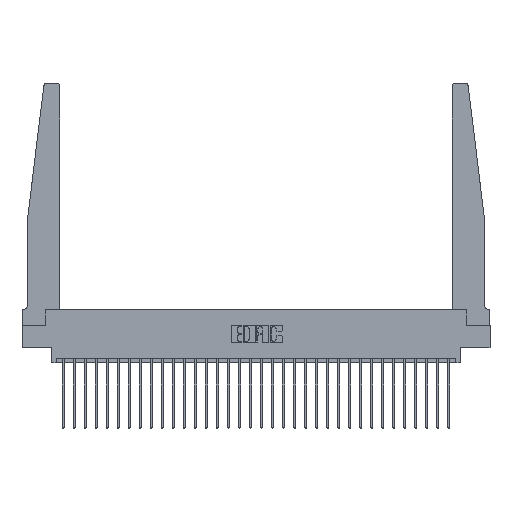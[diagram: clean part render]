
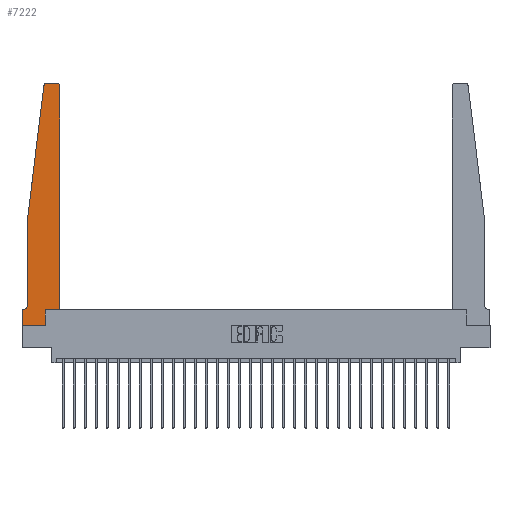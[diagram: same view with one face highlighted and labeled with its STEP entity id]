
A CAD part, top view. The second image highlights one B-rep face of the part: STEP entity #7222.
In plain terms, the highlighted planar face has unit normal (0, 0, 1).
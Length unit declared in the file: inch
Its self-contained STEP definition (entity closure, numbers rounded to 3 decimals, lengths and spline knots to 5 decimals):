
#623 = ORIENTED_EDGE ( 'NONE', *, *, #6422, .T. ) ;
#685 = VERTEX_POINT ( 'NONE', #13505 ) ;
#818 = LINE ( 'NONE', #10123, #12082 ) ;
#1288 = DIRECTION ( 'NONE',  ( 0., -1., 0. ) ) ;
#1533 = ORIENTED_EDGE ( 'NONE', *, *, #24384, .T. ) ;
#1817 = CIRCLE ( 'NONE', #18582, 0.03 ) ;
#1998 = DIRECTION ( 'NONE',  ( 1., 0., 0. ) ) ;
#2332 = LINE ( 'NONE', #20511, #6944 ) ;
#2433 = CARTESIAN_POINT ( 'NONE',  ( 0., 0., 0.37 ) ) ;
#2661 = DIRECTION ( 'NONE',  ( 1., 0., 0. ) ) ;
#2809 = FACE_OUTER_BOUND ( 'NONE', #19211, .T. ) ;
#3032 = CARTESIAN_POINT ( 'NONE',  ( 0.015, 0.1875, 0.37 ) ) ;
#3079 = CARTESIAN_POINT ( 'NONE',  ( 0., 0., 0.37 ) ) ;
#3951 = EDGE_CURVE ( 'NONE', #685, #27609, #2332, .T. ) ;
#4059 = VERTEX_POINT ( 'NONE', #3079 ) ;
#4122 = DIRECTION ( 'NONE',  ( -1., 0., 0. ) ) ;
#5247 = CARTESIAN_POINT ( 'NONE',  ( 0.2605, 0., 0.37 ) ) ;
#5410 = LINE ( 'NONE', #14570, #5514 ) ;
#5513 = VERTEX_POINT ( 'NONE', #26026 ) ;
#5514 = VECTOR ( 'NONE', #23733, 39.37008 ) ;
#5609 = VERTEX_POINT ( 'NONE', #5247 ) ;
#6367 = LINE ( 'NONE', #15544, #20562 ) ;
#6422 = EDGE_CURVE ( 'NONE', #4059, #5609, #15816, .T. ) ;
#6500 = VERTEX_POINT ( 'NONE', #21062 ) ;
#6533 = VERTEX_POINT ( 'NONE', #3032 ) ;
#6812 = CARTESIAN_POINT ( 'NONE',  ( 0.25, 2.75, 0.37 ) ) ;
#6944 = VECTOR ( 'NONE', #13451, 39.37008 ) ;
#6950 = VECTOR ( 'NONE', #1288, 39.37008 ) ;
#7222 = ADVANCED_FACE ( 'NONE', ( #2809 ), #25503, .T. ) ;
#7933 = CARTESIAN_POINT ( 'NONE',  ( 0.2605, 0.18, 0.37 ) ) ;
#7963 = CARTESIAN_POINT ( 'NONE',  ( 0.425, 2.72, 0.37 ) ) ;
#8093 = EDGE_CURVE ( 'NONE', #5513, #685, #28529, .T. ) ;
#8184 = CARTESIAN_POINT ( 'NONE',  ( 0.065, 0.2375, 0.37 ) ) ;
#8297 = EDGE_CURVE ( 'NONE', #27609, #17350, #5410, .T. ) ;
#8595 = DIRECTION ( 'NONE',  ( -1., 0., 0. ) ) ;
#10123 = CARTESIAN_POINT ( 'NONE',  ( 0.425, 0.18, 0.37 ) ) ;
#10318 = ORIENTED_EDGE ( 'NONE', *, *, #13148, .T. ) ;
#10766 = AXIS2_PLACEMENT_3D ( 'NONE', #13682, #22851, #11137 ) ;
#11137 = DIRECTION ( 'NONE',  ( 1., 0., 0. ) ) ;
#11193 = LINE ( 'NONE', #6812, #13063 ) ;
#12082 = VECTOR ( 'NONE', #21400, 39.37008 ) ;
#12377 = ORIENTED_EDGE ( 'NONE', *, *, #8297, .T. ) ;
#12617 = DIRECTION ( 'NONE',  ( 0., 1., 0. ) ) ;
#13063 = VECTOR ( 'NONE', #29522, 39.37008 ) ;
#13087 = ORIENTED_EDGE ( 'NONE', *, *, #17600, .T. ) ;
#13148 = EDGE_CURVE ( 'NONE', #25387, #23842, #818, .T. ) ;
#13277 = DIRECTION ( 'NONE',  ( 1., 0., 0. ) ) ;
#13393 = EDGE_CURVE ( 'NONE', #17350, #6533, #25638, .T. ) ;
#13451 = DIRECTION ( 'NONE',  ( -0.122, -0.992, 0. ) ) ;
#13505 = CARTESIAN_POINT ( 'NONE',  ( 0.24675, 2.72367, 0.37 ) ) ;
#13682 = CARTESIAN_POINT ( 'NONE',  ( 0.27653, 2.72, 0.37 ) ) ;
#13725 = LINE ( 'NONE', #17780, #23103 ) ;
#13769 = EDGE_CURVE ( 'NONE', #5609, #25765, #26892, .T. ) ;
#14570 = CARTESIAN_POINT ( 'NONE',  ( 0.065, 1.25, 0.37 ) ) ;
#15544 = CARTESIAN_POINT ( 'NONE',  ( 0.065, 0.1875, 0.37 ) ) ;
#15816 = LINE ( 'NONE', #2433, #24557 ) ;
#15953 = AXIS2_PLACEMENT_3D ( 'NONE', #23390, #16649, #2661 ) ;
#16202 = EDGE_CURVE ( 'NONE', #6533, #23218, #6367, .T. ) ;
#16649 = DIRECTION ( 'NONE',  ( 0., 0., 1. ) ) ;
#17350 = VERTEX_POINT ( 'NONE', #8184 ) ;
#17600 = EDGE_CURVE ( 'NONE', #6500, #5513, #11193, .T. ) ;
#17780 = CARTESIAN_POINT ( 'NONE',  ( 0.425, 0.18, 0.37 ) ) ;
#18212 = CARTESIAN_POINT ( 'NONE',  ( 0., 0.1875, 0.37 ) ) ;
#18582 = AXIS2_PLACEMENT_3D ( 'NONE', #22870, #23448, #20751 ) ;
#18937 = VECTOR ( 'NONE', #12617, 39.37008 ) ;
#19014 = EDGE_CURVE ( 'NONE', #23218, #4059, #26529, .T. ) ;
#19211 = EDGE_LOOP ( 'NONE', ( #13087, #21166, #28892, #12377, #21195, #19652, #26592, #623, #19559, #1533, #10318, #29486 ) ) ;
#19559 = ORIENTED_EDGE ( 'NONE', *, *, #13769, .T. ) ;
#19652 = ORIENTED_EDGE ( 'NONE', *, *, #16202, .T. ) ;
#20159 = CARTESIAN_POINT ( 'NONE',  ( 0.015, 0.2375, 0.37 ) ) ;
#20410 = CARTESIAN_POINT ( 'NONE',  ( 0.425, 0.18, 0.37 ) ) ;
#20511 = CARTESIAN_POINT ( 'NONE',  ( 0.065, 1.25, 0.37 ) ) ;
#20562 = VECTOR ( 'NONE', #4122, 39.37008 ) ;
#20751 = DIRECTION ( 'NONE',  ( 1., 0., 0. ) ) ;
#21062 = CARTESIAN_POINT ( 'NONE',  ( 0.395, 2.75, 0.37 ) ) ;
#21166 = ORIENTED_EDGE ( 'NONE', *, *, #8093, .T. ) ;
#21195 = ORIENTED_EDGE ( 'NONE', *, *, #13393, .T. ) ;
#21246 = EDGE_CURVE ( 'NONE', #23842, #6500, #1817, .T. ) ;
#21400 = DIRECTION ( 'NONE',  ( 0., 1., 0. ) ) ;
#21428 = CARTESIAN_POINT ( 'NONE',  ( 0., 0., 0.37 ) ) ;
#21606 = CARTESIAN_POINT ( 'NONE',  ( 0.065, 1.25, 0.37 ) ) ;
#22221 = CARTESIAN_POINT ( 'NONE',  ( 0.2605, 0.18, 0.37 ) ) ;
#22851 = DIRECTION ( 'NONE',  ( 0., 0., 1. ) ) ;
#22870 = CARTESIAN_POINT ( 'NONE',  ( 0.395, 2.72, 0.37 ) ) ;
#23103 = VECTOR ( 'NONE', #13277, 39.37008 ) ;
#23218 = VERTEX_POINT ( 'NONE', #18212 ) ;
#23390 = CARTESIAN_POINT ( 'NONE',  ( 0., 0.1875, 0.37 ) ) ;
#23448 = DIRECTION ( 'NONE',  ( 0., 0., 1. ) ) ;
#23733 = DIRECTION ( 'NONE',  ( 0., -1., 0. ) ) ;
#23842 = VERTEX_POINT ( 'NONE', #7963 ) ;
#24384 = EDGE_CURVE ( 'NONE', #25765, #25387, #13725, .T. ) ;
#24557 = VECTOR ( 'NONE', #1998, 39.37008 ) ;
#25387 = VERTEX_POINT ( 'NONE', #20410 ) ;
#25503 = PLANE ( 'NONE',  #15953 ) ;
#25638 = CIRCLE ( 'NONE', #29468, 0.05 ) ;
#25765 = VERTEX_POINT ( 'NONE', #7933 ) ;
#26026 = CARTESIAN_POINT ( 'NONE',  ( 0.27653, 2.75, 0.37 ) ) ;
#26529 = LINE ( 'NONE', #21428, #6950 ) ;
#26592 = ORIENTED_EDGE ( 'NONE', *, *, #19014, .T. ) ;
#26892 = LINE ( 'NONE', #22221, #18937 ) ;
#27609 = VERTEX_POINT ( 'NONE', #21606 ) ;
#28529 = CIRCLE ( 'NONE', #10766, 0.03 ) ;
#28892 = ORIENTED_EDGE ( 'NONE', *, *, #3951, .T. ) ;
#29326 = DIRECTION ( 'NONE',  ( 0., 0., -1. ) ) ;
#29468 = AXIS2_PLACEMENT_3D ( 'NONE', #20159, #29326, #8595 ) ;
#29486 = ORIENTED_EDGE ( 'NONE', *, *, #21246, .T. ) ;
#29522 = DIRECTION ( 'NONE',  ( -1., 0., 0. ) ) ;
